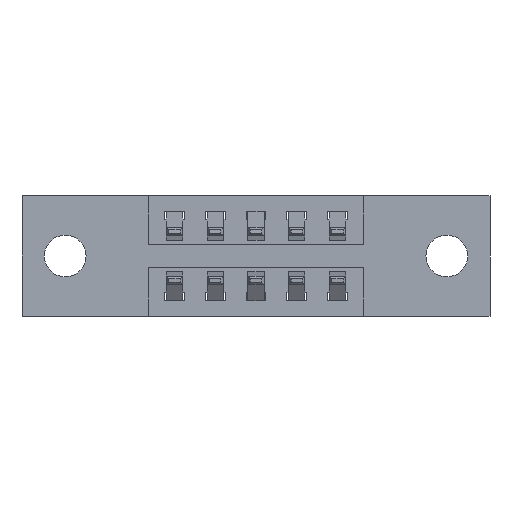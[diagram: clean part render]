
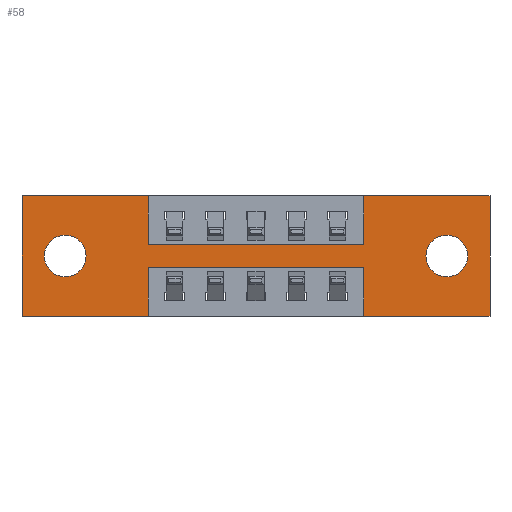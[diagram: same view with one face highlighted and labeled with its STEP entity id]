
A CAD part, front view. The second image highlights one B-rep face of the part: STEP entity #58.
In plain terms, the highlighted planar face has unit normal (0, -1, 0).
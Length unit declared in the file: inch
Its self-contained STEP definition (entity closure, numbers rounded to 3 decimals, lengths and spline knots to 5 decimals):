
#58 = ADVANCED_FACE ( 'NONE', ( #3497, #3639, #3506 ), #4212, .T. ) ;
#65 = DIRECTION ( 'NONE',  ( -1., 0., 0. ) ) ;
#110 = DIRECTION ( 'NONE',  ( 1., 0., 0. ) ) ;
#113 = AXIS2_PLACEMENT_3D ( 'NONE', #5781, #5766, #5751 ) ;
#127 = CARTESIAN_POINT ( 'NONE',  ( 0.3875, 0., -0.15 ) ) ;
#214 = CIRCLE ( 'NONE', #4043, 0.064 ) ;
#375 = DIRECTION ( 'NONE',  ( 0., 0., 1. ) ) ;
#428 = VERTEX_POINT ( 'NONE', #1141 ) ;
#461 = VERTEX_POINT ( 'NONE', #3954 ) ;
#482 = CARTESIAN_POINT ( 'NONE',  ( 0., 0., -0.37 ) ) ;
#528 = CIRCLE ( 'NONE', #113, 0.064 ) ;
#531 = DIRECTION ( 'NONE',  ( 0., 1., 0. ) ) ;
#555 = CARTESIAN_POINT ( 'NONE',  ( 0.1325, 0., -0.185 ) ) ;
#569 = CARTESIAN_POINT ( 'NONE',  ( 1.0475, 0., 0. ) ) ;
#601 = VERTEX_POINT ( 'NONE', #4276 ) ;
#651 = DIRECTION ( 'NONE',  ( 1., 0., 0. ) ) ;
#699 = DIRECTION ( 'NONE',  ( 0., 0., 1. ) ) ;
#719 = VECTOR ( 'NONE', #4871, 39.37008 ) ;
#767 = CARTESIAN_POINT ( 'NONE',  ( 0., 0., -0.37 ) ) ;
#782 = LINE ( 'NONE', #5199, #719 ) ;
#976 = EDGE_CURVE ( 'NONE', #1614, #2402, #8149, .T. ) ;
#1082 = CARTESIAN_POINT ( 'NONE',  ( 0., 0., 0. ) ) ;
#1141 = CARTESIAN_POINT ( 'NONE',  ( 0.3875, 0., 0. ) ) ;
#1183 = VERTEX_POINT ( 'NONE', #6386 ) ;
#1305 = CIRCLE ( 'NONE', #5055, 0.064 ) ;
#1384 = DIRECTION ( 'NONE',  ( -1., 0., 0. ) ) ;
#1478 = CARTESIAN_POINT ( 'NONE',  ( 0.1325, 0., -0.121 ) ) ;
#1537 = DIRECTION ( 'NONE',  ( 0., 0., -1. ) ) ;
#1548 = VECTOR ( 'NONE', #7000, 39.37008 ) ;
#1567 = LINE ( 'NONE', #7460, #1548 ) ;
#1614 = VERTEX_POINT ( 'NONE', #7084 ) ;
#1724 = LINE ( 'NONE', #127, #1892 ) ;
#1811 = CIRCLE ( 'NONE', #7472, 0.064 ) ;
#1817 = VECTOR ( 'NONE', #699, 39.37008 ) ;
#1826 = DIRECTION ( 'NONE',  ( 0., 0., 1. ) ) ;
#1892 = VECTOR ( 'NONE', #110, 39.37008 ) ;
#1936 = LINE ( 'NONE', #569, #1817 ) ;
#1963 = EDGE_CURVE ( 'NONE', #2402, #2799, #5607, .T. ) ;
#2078 = VERTEX_POINT ( 'NONE', #6090 ) ;
#2104 = CARTESIAN_POINT ( 'NONE',  ( 1.435, 0., 0. ) ) ;
#2177 = CARTESIAN_POINT ( 'NONE',  ( 1.0475, 0., -0.37 ) ) ;
#2180 = DIRECTION ( 'NONE',  ( 1., 0., 0. ) ) ;
#2306 = VECTOR ( 'NONE', #1826, 39.37008 ) ;
#2320 = EDGE_CURVE ( 'NONE', #3928, #428, #4369, .T. ) ;
#2324 = EDGE_CURVE ( 'NONE', #7585, #4414, #4219, .T. ) ;
#2401 = VECTOR ( 'NONE', #2180, 39.37008 ) ;
#2402 = VERTEX_POINT ( 'NONE', #6301 ) ;
#2418 = CARTESIAN_POINT ( 'NONE',  ( 0., 0., 0. ) ) ;
#2484 = LINE ( 'NONE', #2418, #2401 ) ;
#2641 = LINE ( 'NONE', #2177, #2306 ) ;
#2756 = EDGE_CURVE ( 'NONE', #2078, #1614, #2484, .T. ) ;
#2799 = VERTEX_POINT ( 'NONE', #8260 ) ;
#2830 = DIRECTION ( 'NONE',  ( -1., 0., 0. ) ) ;
#2899 = CARTESIAN_POINT ( 'NONE',  ( 0.3875, 0., -0.22 ) ) ;
#2932 = EDGE_CURVE ( 'NONE', #1183, #4249, #1811, .T. ) ;
#3057 = CARTESIAN_POINT ( 'NONE',  ( 0., 0., 0. ) ) ;
#3099 = EDGE_CURVE ( 'NONE', #5247, #461, #1305, .T. ) ;
#3251 = DIRECTION ( 'NONE',  ( 0., 0., -1. ) ) ;
#3287 = DIRECTION ( 'NONE',  ( 0., 0., -1. ) ) ;
#3295 = EDGE_CURVE ( 'NONE', #4414, #3928, #782, .T. ) ;
#3364 = VECTOR ( 'NONE', #2830, 39.37008 ) ;
#3397 = CARTESIAN_POINT ( 'NONE',  ( 0.3875, 0., -0.37 ) ) ;
#3398 = LINE ( 'NONE', #2899, #3364 ) ;
#3497 = FACE_BOUND ( 'NONE', #3938, .T. ) ;
#3506 = FACE_OUTER_BOUND ( 'NONE', #5626, .T. ) ;
#3528 = VECTOR ( 'NONE', #3251, 39.37008 ) ;
#3550 = LINE ( 'NONE', #3397, #3528 ) ;
#3639 = FACE_BOUND ( 'NONE', #3908, .T. ) ;
#3908 = EDGE_LOOP ( 'NONE', ( #6568, #6590 ) ) ;
#3928 = VERTEX_POINT ( 'NONE', #1082 ) ;
#3938 = EDGE_LOOP ( 'NONE', ( #6510, #6561 ) ) ;
#3948 = AXIS2_PLACEMENT_3D ( 'NONE', #4757, #4309, #1537 ) ;
#3954 = CARTESIAN_POINT ( 'NONE',  ( 0.1325, 0., -0.249 ) ) ;
#3970 = VERTEX_POINT ( 'NONE', #7258 ) ;
#4043 = AXIS2_PLACEMENT_3D ( 'NONE', #5166, #5155, #5129 ) ;
#4100 = VERTEX_POINT ( 'NONE', #7765 ) ;
#4159 = VECTOR ( 'NONE', #65, 39.37008 ) ;
#4194 = VECTOR ( 'NONE', #651, 39.37008 ) ;
#4212 = PLANE ( 'NONE',  #3948 ) ;
#4219 = LINE ( 'NONE', #482, #4159 ) ;
#4249 = VERTEX_POINT ( 'NONE', #6646 ) ;
#4276 = CARTESIAN_POINT ( 'NONE',  ( 0.3875, 0., -0.15 ) ) ;
#4309 = DIRECTION ( 'NONE',  ( 0., -1., 0. ) ) ;
#4369 = LINE ( 'NONE', #3057, #4194 ) ;
#4414 = VERTEX_POINT ( 'NONE', #5576 ) ;
#4649 = EDGE_CURVE ( 'NONE', #3970, #7585, #3550, .T. ) ;
#4670 = CARTESIAN_POINT ( 'NONE',  ( 0.3875, 0., -0.37 ) ) ;
#4683 = EDGE_CURVE ( 'NONE', #7430, #3970, #3398, .T. ) ;
#4717 = DIRECTION ( 'NONE',  ( 0., 0., -1. ) ) ;
#4737 = DIRECTION ( 'NONE',  ( 0., 1., 0. ) ) ;
#4757 = CARTESIAN_POINT ( 'NONE',  ( 0., 0., -0.37 ) ) ;
#4803 = CARTESIAN_POINT ( 'NONE',  ( 1.3025, 0., -0.185 ) ) ;
#4808 = EDGE_CURVE ( 'NONE', #2799, #7430, #2641, .T. ) ;
#4871 = DIRECTION ( 'NONE',  ( 0., 0., 1. ) ) ;
#4909 = EDGE_CURVE ( 'NONE', #4100, #2078, #1936, .T. ) ;
#4937 = EDGE_CURVE ( 'NONE', #601, #4100, #1724, .T. ) ;
#4977 = EDGE_CURVE ( 'NONE', #428, #601, #1567, .T. ) ;
#5055 = AXIS2_PLACEMENT_3D ( 'NONE', #555, #531, #375 ) ;
#5129 = DIRECTION ( 'NONE',  ( 0., 0., 1. ) ) ;
#5155 = DIRECTION ( 'NONE',  ( 0., 1., 0. ) ) ;
#5166 = CARTESIAN_POINT ( 'NONE',  ( 0.1325, 0., -0.185 ) ) ;
#5199 = CARTESIAN_POINT ( 'NONE',  ( 0., 0., 0. ) ) ;
#5247 = VERTEX_POINT ( 'NONE', #1478 ) ;
#5476 = VECTOR ( 'NONE', #1384, 39.37008 ) ;
#5564 = CARTESIAN_POINT ( 'NONE',  ( 1.0475, 0., -0.22 ) ) ;
#5576 = CARTESIAN_POINT ( 'NONE',  ( 0., 0., -0.37 ) ) ;
#5607 = LINE ( 'NONE', #767, #5476 ) ;
#5626 = EDGE_LOOP ( 'NONE', ( #6608, #6663, #6680, #6686, #6708, #6729, #6736, #6761, #6784, #6793, #6819, #6832 ) ) ;
#5751 = DIRECTION ( 'NONE',  ( 0., 0., -1. ) ) ;
#5766 = DIRECTION ( 'NONE',  ( 0., 1., 0. ) ) ;
#5781 = CARTESIAN_POINT ( 'NONE',  ( 1.3025, 0., -0.185 ) ) ;
#6090 = CARTESIAN_POINT ( 'NONE',  ( 1.0475, 0., 0. ) ) ;
#6292 = VECTOR ( 'NONE', #3287, 39.37008 ) ;
#6301 = CARTESIAN_POINT ( 'NONE',  ( 1.435, 0., -0.37 ) ) ;
#6386 = CARTESIAN_POINT ( 'NONE',  ( 1.3025, 0., -0.121 ) ) ;
#6510 = ORIENTED_EDGE ( 'NONE', *, *, #2932, .T. ) ;
#6561 = ORIENTED_EDGE ( 'NONE', *, *, #7340, .T. ) ;
#6568 = ORIENTED_EDGE ( 'NONE', *, *, #3099, .T. ) ;
#6590 = ORIENTED_EDGE ( 'NONE', *, *, #7468, .T. ) ;
#6608 = ORIENTED_EDGE ( 'NONE', *, *, #4649, .F. ) ;
#6646 = CARTESIAN_POINT ( 'NONE',  ( 1.3025, 0., -0.249 ) ) ;
#6663 = ORIENTED_EDGE ( 'NONE', *, *, #4683, .F. ) ;
#6680 = ORIENTED_EDGE ( 'NONE', *, *, #4808, .F. ) ;
#6686 = ORIENTED_EDGE ( 'NONE', *, *, #1963, .F. ) ;
#6708 = ORIENTED_EDGE ( 'NONE', *, *, #976, .F. ) ;
#6729 = ORIENTED_EDGE ( 'NONE', *, *, #2756, .F. ) ;
#6736 = ORIENTED_EDGE ( 'NONE', *, *, #4909, .F. ) ;
#6761 = ORIENTED_EDGE ( 'NONE', *, *, #4937, .F. ) ;
#6784 = ORIENTED_EDGE ( 'NONE', *, *, #4977, .F. ) ;
#6793 = ORIENTED_EDGE ( 'NONE', *, *, #2320, .F. ) ;
#6819 = ORIENTED_EDGE ( 'NONE', *, *, #3295, .F. ) ;
#6832 = ORIENTED_EDGE ( 'NONE', *, *, #2324, .F. ) ;
#7000 = DIRECTION ( 'NONE',  ( 0., 0., -1. ) ) ;
#7084 = CARTESIAN_POINT ( 'NONE',  ( 1.435, 0., 0. ) ) ;
#7258 = CARTESIAN_POINT ( 'NONE',  ( 0.3875, 0., -0.22 ) ) ;
#7340 = EDGE_CURVE ( 'NONE', #4249, #1183, #528, .T. ) ;
#7430 = VERTEX_POINT ( 'NONE', #5564 ) ;
#7460 = CARTESIAN_POINT ( 'NONE',  ( 0.3875, 0., 0. ) ) ;
#7468 = EDGE_CURVE ( 'NONE', #461, #5247, #214, .T. ) ;
#7472 = AXIS2_PLACEMENT_3D ( 'NONE', #4803, #4737, #4717 ) ;
#7585 = VERTEX_POINT ( 'NONE', #4670 ) ;
#7765 = CARTESIAN_POINT ( 'NONE',  ( 1.0475, 0., -0.15 ) ) ;
#8149 = LINE ( 'NONE', #2104, #6292 ) ;
#8260 = CARTESIAN_POINT ( 'NONE',  ( 1.0475, 0., -0.37 ) ) ;
